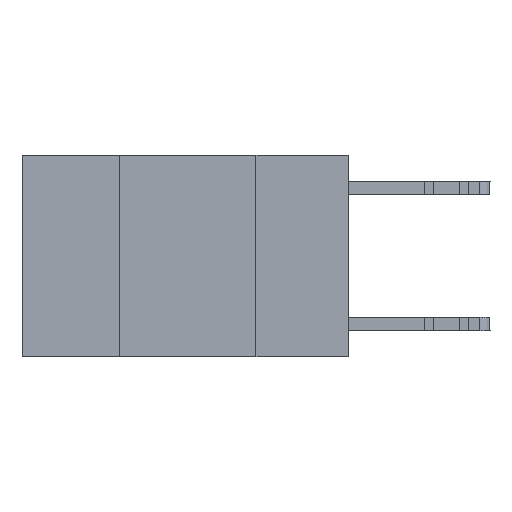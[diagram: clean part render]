
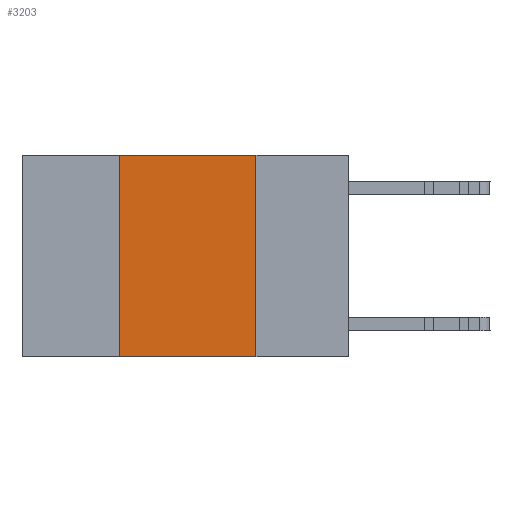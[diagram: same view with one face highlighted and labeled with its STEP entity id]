
A CAD part, left-side view. The second image highlights one B-rep face of the part: STEP entity #3203.
In plain terms, the highlighted planar face has unit normal (-1, 0, 0).
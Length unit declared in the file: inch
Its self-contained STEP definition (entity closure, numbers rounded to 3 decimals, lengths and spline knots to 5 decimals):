
#2453 = DIRECTION ( 'NONE',  ( 0., -1., 0. ) ) ;
#3191 = DIRECTION ( 'NONE',  ( 0., -1., 0. ) ) ;
#3203 = ADVANCED_FACE ( 'NONE', ( #3258 ), #13957, .F. ) ;
#3258 = FACE_OUTER_BOUND ( 'NONE', #23688, .T. ) ;
#5140 = DIRECTION ( 'NONE',  ( 0., 0., -1. ) ) ;
#5571 = CARTESIAN_POINT ( 'NONE',  ( 0., 0.42, 0. ) ) ;
#6682 = LINE ( 'NONE', #9033, #14721 ) ;
#6767 = ORIENTED_EDGE ( 'NONE', *, *, #12264, .F. ) ;
#7172 = LINE ( 'NONE', #25138, #7442 ) ;
#7280 = LINE ( 'NONE', #24940, #11262 ) ;
#7442 = VECTOR ( 'NONE', #5140, 39.37008 ) ;
#7644 = DIRECTION ( 'NONE',  ( 0., 0., -1. ) ) ;
#8334 = CARTESIAN_POINT ( 'NONE',  ( 0., 0.42, -0.37 ) ) ;
#8796 = ORIENTED_EDGE ( 'NONE', *, *, #12384, .F. ) ;
#9033 = CARTESIAN_POINT ( 'NONE',  ( 0., 0.6, -0.37 ) ) ;
#9669 = EDGE_CURVE ( 'NONE', #26391, #24810, #6682, .T. ) ;
#9690 = CARTESIAN_POINT ( 'NONE',  ( 0., 0.6, 0. ) ) ;
#9983 = DIRECTION ( 'NONE',  ( 1., 0., 0. ) ) ;
#11262 = VECTOR ( 'NONE', #3191, 39.37008 ) ;
#12264 = EDGE_CURVE ( 'NONE', #21201, #24810, #7172, .T. ) ;
#12384 = EDGE_CURVE ( 'NONE', #26391, #25131, #25707, .T. ) ;
#12620 = ORIENTED_EDGE ( 'NONE', *, *, #12676, .F. ) ;
#12676 = EDGE_CURVE ( 'NONE', #25131, #21201, #7280, .T. ) ;
#13957 = PLANE ( 'NONE',  #23717 ) ;
#14721 = VECTOR ( 'NONE', #2453, 39.37008 ) ;
#14965 = VECTOR ( 'NONE', #23494, 39.37008 ) ;
#16142 = CARTESIAN_POINT ( 'NONE',  ( 0., 0.17, 0. ) ) ;
#21198 = CARTESIAN_POINT ( 'NONE',  ( 0., 0.42, 0. ) ) ;
#21201 = VERTEX_POINT ( 'NONE', #16142 ) ;
#22113 = CARTESIAN_POINT ( 'NONE',  ( 0., 0.17, -0.37 ) ) ;
#22258 = ORIENTED_EDGE ( 'NONE', *, *, #9669, .T. ) ;
#23494 = DIRECTION ( 'NONE',  ( 0., 0., 1. ) ) ;
#23688 = EDGE_LOOP ( 'NONE', ( #6767, #12620, #8796, #22258 ) ) ;
#23717 = AXIS2_PLACEMENT_3D ( 'NONE', #9690, #9983, #7644 ) ;
#24810 = VERTEX_POINT ( 'NONE', #22113 ) ;
#24940 = CARTESIAN_POINT ( 'NONE',  ( 0., 0.6, 0. ) ) ;
#25131 = VERTEX_POINT ( 'NONE', #21198 ) ;
#25138 = CARTESIAN_POINT ( 'NONE',  ( 0., 0.17, 0. ) ) ;
#25707 = LINE ( 'NONE', #5571, #14965 ) ;
#26391 = VERTEX_POINT ( 'NONE', #8334 ) ;
